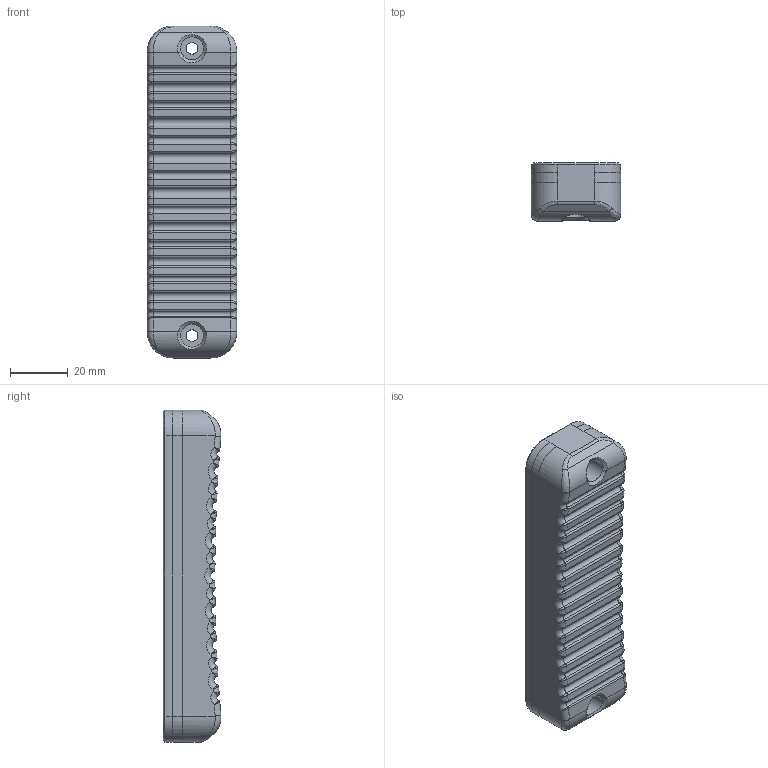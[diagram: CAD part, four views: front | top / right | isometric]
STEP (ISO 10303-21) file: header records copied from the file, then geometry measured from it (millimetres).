
FILE_DESCRIPTION(/* description */ (''),/* implementation_level */ '2;1');
FILE_NAME(/* name */ 'Concave Buttpad.step',/* time_stamp */ '2021-07-28T09:03:03-04:00',/* author */ (''),/* organization */ (''),/* preprocessor_version */ 'ST-DEVELOPER v18.1',/* originating_system */ 'Autodesk Translation Framework v10.9.0.1377',/* authorisation */ '');
FILE_SCHEMA (('AUTOMOTIVE_DESIGN { 1 0 10303 214 3 1 1 }'));
Length unit declared in the file: millimetre
Products named in the file (1): Concave Buttpad
Bounding box: 31 x 20.09 x 115 mm (x, y, z)
Volume: 62151.5 mm3; surface area: 12867.4 mm2
Topology: 1 solids, 1 shells, 250 faces, 586 edges, 278 vertices
Faces by surface type: bspline 84, cylinder 77, torus 74, plane 13, cone 2
Full cylindrical faces by diameter (mm): 4 x2, 8 x2
Entity records: 10508 total; most frequent: CARTESIAN_POINT 5597, ORIENTED_EDGE 1052, DIRECTION 946, EDGE_CURVE 526, AXIS2_PLACEMENT_3D 415, VERTEX_POINT 278, EDGE_LOOP 254, FACE_OUTER_BOUND 250
